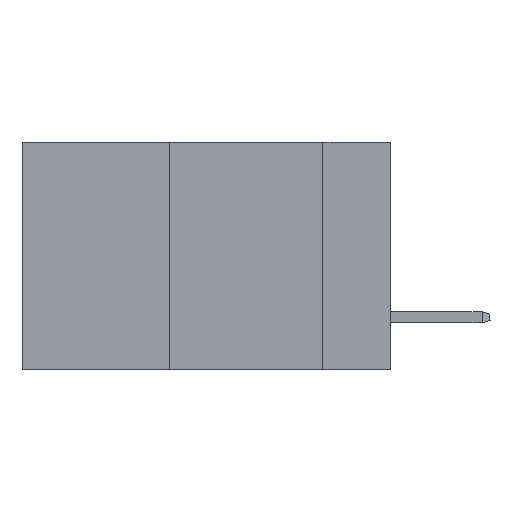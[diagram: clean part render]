
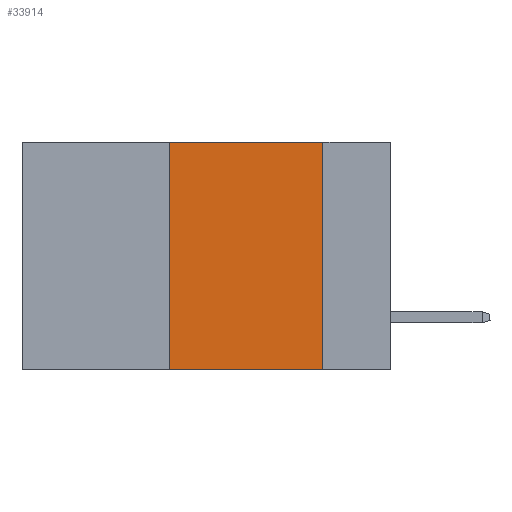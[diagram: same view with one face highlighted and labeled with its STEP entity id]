
A CAD part, left-side view. The second image highlights one B-rep face of the part: STEP entity #33914.
In plain terms, the highlighted planar face has unit normal (-1, 0, 0).
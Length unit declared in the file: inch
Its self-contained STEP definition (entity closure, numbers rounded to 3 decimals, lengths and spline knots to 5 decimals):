
#1453 = CARTESIAN_POINT ( 'NONE',  ( 0., 0.11, 0. ) ) ;
#2879 = ORIENTED_EDGE ( 'NONE', *, *, #7777, .F. ) ;
#7777 = EDGE_CURVE ( 'NONE', #13191, #26192, #12329, .T. ) ;
#9215 = CARTESIAN_POINT ( 'NONE',  ( 0., 0.6, -0.37 ) ) ;
#12024 = DIRECTION ( 'NONE',  ( 0., 0., -1. ) ) ;
#12129 = FACE_OUTER_BOUND ( 'NONE', #18946, .T. ) ;
#12263 = EDGE_CURVE ( 'NONE', #43213, #13191, #29801, .T. ) ;
#12329 = LINE ( 'NONE', #1453, #33986 ) ;
#13191 = VERTEX_POINT ( 'NONE', #45315 ) ;
#15573 = CARTESIAN_POINT ( 'NONE',  ( 0., 0.6, 0. ) ) ;
#15835 = LINE ( 'NONE', #31736, #24717 ) ;
#16640 = LINE ( 'NONE', #9215, #27697 ) ;
#18523 = ORIENTED_EDGE ( 'NONE', *, *, #44245, .T. ) ;
#18604 = ORIENTED_EDGE ( 'NONE', *, *, #12263, .F. ) ;
#18946 = EDGE_LOOP ( 'NONE', ( #2879, #18604, #24961, #18523 ) ) ;
#19211 = CARTESIAN_POINT ( 'NONE',  ( 0., 0.6, 0. ) ) ;
#21514 = VECTOR ( 'NONE', #22654, 39.37008 ) ;
#22654 = DIRECTION ( 'NONE',  ( 0., -1., 0. ) ) ;
#24584 = CARTESIAN_POINT ( 'NONE',  ( 0., 0.36, 0. ) ) ;
#24717 = VECTOR ( 'NONE', #31587, 39.37008 ) ;
#24961 = ORIENTED_EDGE ( 'NONE', *, *, #41204, .F. ) ;
#25857 = AXIS2_PLACEMENT_3D ( 'NONE', #15573, #40410, #43986 ) ;
#26192 = VERTEX_POINT ( 'NONE', #41981 ) ;
#26586 = DIRECTION ( 'NONE',  ( 0., -1., 0. ) ) ;
#27697 = VECTOR ( 'NONE', #26586, 39.37008 ) ;
#29801 = LINE ( 'NONE', #19211, #21514 ) ;
#31587 = DIRECTION ( 'NONE',  ( 0., 0., 1. ) ) ;
#31736 = CARTESIAN_POINT ( 'NONE',  ( 0., 0.36, 0. ) ) ;
#33914 = ADVANCED_FACE ( 'NONE', ( #12129 ), #44134, .F. ) ;
#33986 = VECTOR ( 'NONE', #12024, 39.37008 ) ;
#35256 = CARTESIAN_POINT ( 'NONE',  ( 0., 0.36, -0.37 ) ) ;
#40410 = DIRECTION ( 'NONE',  ( 1., 0., 0. ) ) ;
#41204 = EDGE_CURVE ( 'NONE', #41999, #43213, #15835, .T. ) ;
#41981 = CARTESIAN_POINT ( 'NONE',  ( 0., 0.11, -0.37 ) ) ;
#41999 = VERTEX_POINT ( 'NONE', #35256 ) ;
#43213 = VERTEX_POINT ( 'NONE', #24584 ) ;
#43986 = DIRECTION ( 'NONE',  ( 0., 0., -1. ) ) ;
#44134 = PLANE ( 'NONE',  #25857 ) ;
#44245 = EDGE_CURVE ( 'NONE', #41999, #26192, #16640, .T. ) ;
#45315 = CARTESIAN_POINT ( 'NONE',  ( 0., 0.11, 0. ) ) ;
